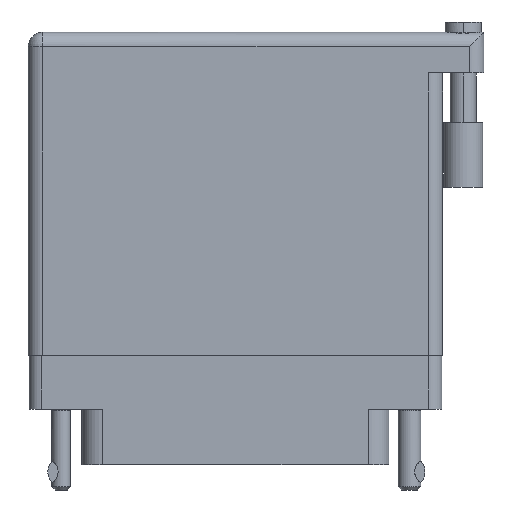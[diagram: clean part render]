
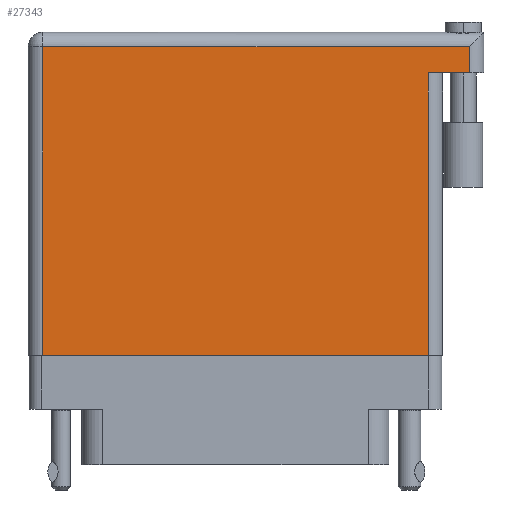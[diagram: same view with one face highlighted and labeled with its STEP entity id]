
A CAD part, front view. The second image highlights one B-rep face of the part: STEP entity #27343.
In plain terms, the highlighted face is planar.
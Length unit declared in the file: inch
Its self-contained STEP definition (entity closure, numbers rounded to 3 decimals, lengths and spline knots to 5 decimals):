
#1459 = ORIENTED_EDGE ( 'NONE', *, *, #28940, .T. ) ;
#3487 = LINE ( 'NONE', #44448, #39317 ) ;
#3524 = DIRECTION ( 'NONE',  ( 0., -1., 0. ) ) ;
#7235 = CARTESIAN_POINT ( 'NONE',  ( 2.138, 1.369, 0. ) ) ;
#8781 = CARTESIAN_POINT ( 'NONE',  ( 1.938, 0., 0. ) ) ;
#9132 = ORIENTED_EDGE ( 'NONE', *, *, #41981, .T. ) ;
#11085 = CARTESIAN_POINT ( 'NONE',  ( 0., 1.496, 0. ) ) ;
#11554 = LINE ( 'NONE', #26505, #25972 ) ;
#11775 = DIRECTION ( 'NONE',  ( 0., 0., -1. ) ) ;
#11883 = EDGE_CURVE ( 'NONE', #43937, #47290, #44295, .T. ) ;
#12410 = VECTOR ( 'NONE', #25733, 39.37008 ) ;
#13332 = ORIENTED_EDGE ( 'NONE', *, *, #11883, .T. ) ;
#13771 = EDGE_LOOP ( 'NONE', ( #32066, #13332, #31256, #9132, #21922, #1459 ) ) ;
#14915 = DIRECTION ( 'NONE',  ( -1., 0., 0. ) ) ;
#15708 = EDGE_CURVE ( 'NONE', #16908, #17024, #27404, .T. ) ;
#16225 = LINE ( 'NONE', #20236, #43341 ) ;
#16500 = CARTESIAN_POINT ( 'NONE',  ( 0.07, 1.496, 0. ) ) ;
#16562 = CARTESIAN_POINT ( 'NONE',  ( 0.07, 0., 0. ) ) ;
#16908 = VERTEX_POINT ( 'NONE', #23407 ) ;
#17024 = VERTEX_POINT ( 'NONE', #16500 ) ;
#18541 = EDGE_CURVE ( 'NONE', #26294, #43937, #16225, .T. ) ;
#19201 = CARTESIAN_POINT ( 'NONE',  ( 0., 1.566, 0. ) ) ;
#19351 = DIRECTION ( 'NONE',  ( -1., 0., 0. ) ) ;
#19791 = EDGE_CURVE ( 'NONE', #33527, #47290, #11554, .T. ) ;
#20236 = CARTESIAN_POINT ( 'NONE',  ( 0., 0., 0. ) ) ;
#20666 = VECTOR ( 'NONE', #26949, 39.37008 ) ;
#21922 = ORIENTED_EDGE ( 'NONE', *, *, #15708, .T. ) ;
#22237 = PLANE ( 'NONE',  #43954 ) ;
#22637 = DIRECTION ( 'NONE',  ( 0., 1., 0. ) ) ;
#23407 = CARTESIAN_POINT ( 'NONE',  ( 2.138, 1.496, 0. ) ) ;
#25733 = DIRECTION ( 'NONE',  ( -1., 0., 0. ) ) ;
#25972 = VECTOR ( 'NONE', #14915, 39.37008 ) ;
#26173 = VECTOR ( 'NONE', #3524, 39.37008 ) ;
#26294 = VERTEX_POINT ( 'NONE', #16562 ) ;
#26505 = CARTESIAN_POINT ( 'NONE',  ( 2.208, 1.369, 0. ) ) ;
#26949 = DIRECTION ( 'NONE',  ( 0., 1., 0. ) ) ;
#27343 = ADVANCED_FACE ( 'NONE', ( #34935 ), #22237, .F. ) ;
#27404 = LINE ( 'NONE', #11085, #12410 ) ;
#28940 = EDGE_CURVE ( 'NONE', #17024, #26294, #44089, .T. ) ;
#31256 = ORIENTED_EDGE ( 'NONE', *, *, #19791, .F. ) ;
#32066 = ORIENTED_EDGE ( 'NONE', *, *, #18541, .T. ) ;
#32783 = CARTESIAN_POINT ( 'NONE',  ( 0.07, 0., 0. ) ) ;
#33527 = VERTEX_POINT ( 'NONE', #7235 ) ;
#33573 = CARTESIAN_POINT ( 'NONE',  ( 1.938, 1.369, 0. ) ) ;
#34568 = DIRECTION ( 'NONE',  ( 1., 0., 0. ) ) ;
#34935 = FACE_OUTER_BOUND ( 'NONE', #13771, .T. ) ;
#39317 = VECTOR ( 'NONE', #22637, 39.37008 ) ;
#41981 = EDGE_CURVE ( 'NONE', #33527, #16908, #3487, .T. ) ;
#43341 = VECTOR ( 'NONE', #34568, 39.37008 ) ;
#43937 = VERTEX_POINT ( 'NONE', #8781 ) ;
#43954 = AXIS2_PLACEMENT_3D ( 'NONE', #19201, #11775, #19351 ) ;
#44089 = LINE ( 'NONE', #32783, #26173 ) ;
#44295 = LINE ( 'NONE', #33573, #20666 ) ;
#44448 = CARTESIAN_POINT ( 'NONE',  ( 2.138, 1.566, 0. ) ) ;
#47096 = CARTESIAN_POINT ( 'NONE',  ( 1.938, 1.369, 0. ) ) ;
#47290 = VERTEX_POINT ( 'NONE', #47096 ) ;
